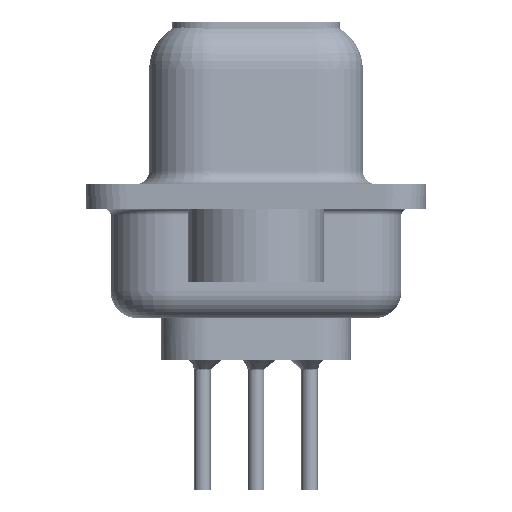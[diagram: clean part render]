
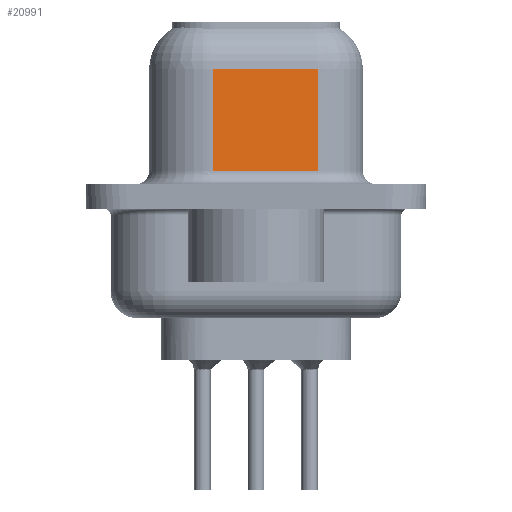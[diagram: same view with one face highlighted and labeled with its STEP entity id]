
A CAD part, left-side view. The second image highlights one B-rep face of the part: STEP entity #20991.
In plain terms, the highlighted planar face has unit normal (-0.985, -0.174, 0).
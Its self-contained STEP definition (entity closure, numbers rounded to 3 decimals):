
#1344 = CARTESIAN_POINT ( 'NONE',  ( 5.038, -2.297, 0.95 ) ) ;
#1386 = CARTESIAN_POINT ( 'NONE',  ( 5.038, -2.297, 6.45 ) ) ;
#3304 = AXIS2_PLACEMENT_3D ( 'NONE', #1386, #8460, #32546 ) ;
#3584 = VECTOR ( 'NONE', #32756, 1000. ) ;
#3879 = DIRECTION ( 'NONE',  ( 0., 0., -1. ) ) ;
#4396 = PLANE ( 'NONE',  #3304 ) ;
#5378 = LINE ( 'NONE', #14858, #25105 ) ;
#6752 = ORIENTED_EDGE ( 'NONE', *, *, #11049, .T. ) ;
#7023 = ORIENTED_EDGE ( 'NONE', *, *, #17712, .T. ) ;
#8460 = DIRECTION ( 'NONE',  ( 0.985, 0.174, 0. ) ) ;
#9165 = VERTEX_POINT ( 'NONE', #37001 ) ;
#11049 = EDGE_CURVE ( 'NONE', #34291, #17571, #11053, .T. ) ;
#11053 = LINE ( 'NONE', #1344, #16715 ) ;
#11452 = DIRECTION ( 'NONE',  ( -0.174, 0.985, 0. ) ) ;
#11512 = LINE ( 'NONE', #13726, #3584 ) ;
#11773 = VECTOR ( 'NONE', #3879, 1000. ) ;
#13726 = CARTESIAN_POINT ( 'NONE',  ( 5.038, -2.297, 6.45 ) ) ;
#13962 = CARTESIAN_POINT ( 'NONE',  ( 4.35, 1.603, 6.45 ) ) ;
#14858 = CARTESIAN_POINT ( 'NONE',  ( 5.038, -2.297, 4.7 ) ) ;
#15656 = CARTESIAN_POINT ( 'NONE',  ( 4.35, 1.603, 0.95 ) ) ;
#16715 = VECTOR ( 'NONE', #35711, 1000. ) ;
#17571 = VERTEX_POINT ( 'NONE', #34937 ) ;
#17712 = EDGE_CURVE ( 'NONE', #19131, #9165, #5378, .T. ) ;
#19131 = VERTEX_POINT ( 'NONE', #27955 ) ;
#19665 = ORIENTED_EDGE ( 'NONE', *, *, #23564, .T. ) ;
#20358 = FACE_OUTER_BOUND ( 'NONE', #28499, .T. ) ;
#20991 = ADVANCED_FACE ( 'NONE', ( #20358 ), #4396, .F. ) ;
#23564 = EDGE_CURVE ( 'NONE', #9165, #34291, #26321, .T. ) ;
#25105 = VECTOR ( 'NONE', #11452, 1000. ) ;
#25127 = ORIENTED_EDGE ( 'NONE', *, *, #26907, .F. ) ;
#26321 = LINE ( 'NONE', #13962, #11773 ) ;
#26907 = EDGE_CURVE ( 'NONE', #19131, #17571, #11512, .T. ) ;
#27955 = CARTESIAN_POINT ( 'NONE',  ( 5.038, -2.297, 4.7 ) ) ;
#28499 = EDGE_LOOP ( 'NONE', ( #25127, #7023, #19665, #6752 ) ) ;
#32546 = DIRECTION ( 'NONE',  ( -0.174, 0.985, 0. ) ) ;
#32756 = DIRECTION ( 'NONE',  ( 0., 0., -1. ) ) ;
#34291 = VERTEX_POINT ( 'NONE', #15656 ) ;
#34937 = CARTESIAN_POINT ( 'NONE',  ( 5.038, -2.297, 0.95 ) ) ;
#35711 = DIRECTION ( 'NONE',  ( 0.174, -0.985, 0. ) ) ;
#37001 = CARTESIAN_POINT ( 'NONE',  ( 4.35, 1.603, 4.7 ) ) ;
